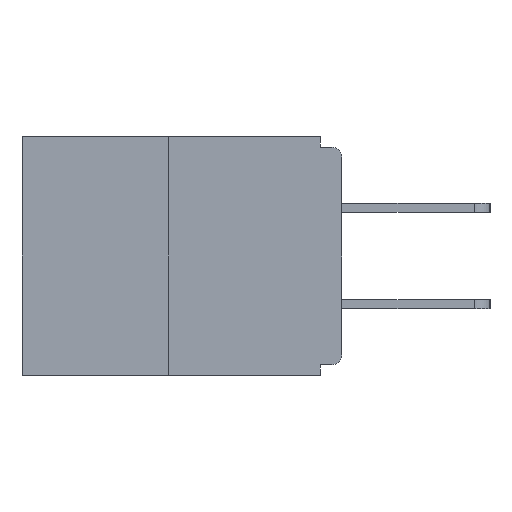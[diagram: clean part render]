
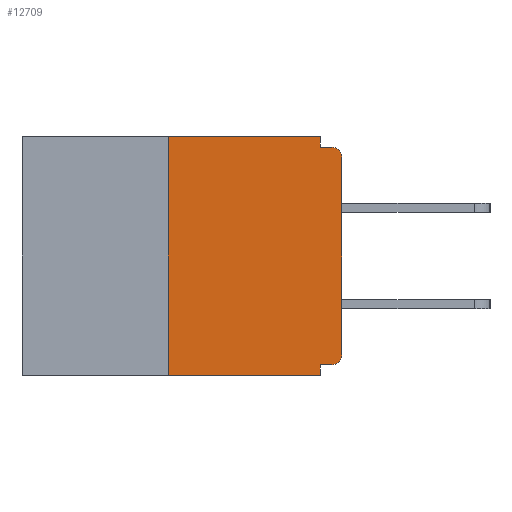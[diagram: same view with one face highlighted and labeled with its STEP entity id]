
A CAD part, left-side view. The second image highlights one B-rep face of the part: STEP entity #12709.
In plain terms, the highlighted planar face has unit normal (-1, 0, 0).
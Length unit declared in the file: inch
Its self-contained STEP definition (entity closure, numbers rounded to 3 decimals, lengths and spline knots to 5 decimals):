
#410 = VERTEX_POINT ( 'NONE', #9253 ) ;
#653 = CARTESIAN_POINT ( 'NONE',  ( 0., 0.25, 0. ) ) ;
#848 = CARTESIAN_POINT ( 'NONE',  ( 0., 0.031, -0.328 ) ) ;
#2643 = DIRECTION ( 'NONE',  ( 0., 0., 1. ) ) ;
#3361 = CARTESIAN_POINT ( 'NONE',  ( 0., 0.25, -0.343 ) ) ;
#3459 = CARTESIAN_POINT ( 'NONE',  ( 0., 0.46, 0. ) ) ;
#4541 = CARTESIAN_POINT ( 'NONE',  ( 0., 0.015, -0.03 ) ) ;
#4756 = CARTESIAN_POINT ( 'NONE',  ( 0., 0., -0.03 ) ) ;
#5009 = EDGE_CURVE ( 'NONE', #21462, #10018, #9504, .T. ) ;
#5322 = LINE ( 'NONE', #5993, #16218 ) ;
#5693 = CARTESIAN_POINT ( 'NONE',  ( 0., 0.031, 0. ) ) ;
#5720 = VERTEX_POINT ( 'NONE', #5693 ) ;
#5853 = DIRECTION ( 'NONE',  ( 0., 0., -1. ) ) ;
#5993 = CARTESIAN_POINT ( 'NONE',  ( 0., 0.031, -0.343 ) ) ;
#6022 = LINE ( 'NONE', #8962, #7115 ) ;
#6177 = LINE ( 'NONE', #7917, #17413 ) ;
#6811 = VERTEX_POINT ( 'NONE', #17372 ) ;
#6872 = EDGE_CURVE ( 'NONE', #9885, #410, #14978, .T. ) ;
#7115 = VECTOR ( 'NONE', #2643, 39.37008 ) ;
#7177 = ORIENTED_EDGE ( 'NONE', *, *, #23839, .T. ) ;
#7222 = ORIENTED_EDGE ( 'NONE', *, *, #8979, .F. ) ;
#7246 = CARTESIAN_POINT ( 'NONE',  ( 0., 0., -0.015 ) ) ;
#7917 = CARTESIAN_POINT ( 'NONE',  ( 0., 0.031, 0. ) ) ;
#8712 = VECTOR ( 'NONE', #20625, 39.37008 ) ;
#8740 = CIRCLE ( 'NONE', #18143, 0.015 ) ;
#8849 = DIRECTION ( 'NONE',  ( 0., -1., 0. ) ) ;
#8962 = CARTESIAN_POINT ( 'NONE',  ( 0., 0.25, 0. ) ) ;
#8979 = EDGE_CURVE ( 'NONE', #28953, #5720, #11420, .T. ) ;
#9055 = DIRECTION ( 'NONE',  ( 0., 0., -1. ) ) ;
#9080 = DIRECTION ( 'NONE',  ( -1., 0., 0. ) ) ;
#9253 = CARTESIAN_POINT ( 'NONE',  ( 0., 0.031, -0.343 ) ) ;
#9504 = CIRCLE ( 'NONE', #20768, 0.015 ) ;
#9885 = VERTEX_POINT ( 'NONE', #3361 ) ;
#10018 = VERTEX_POINT ( 'NONE', #20352 ) ;
#10610 = EDGE_LOOP ( 'NONE', ( #7222, #22445, #24540, #17256, #17356, #27365, #7177, #24020, #20868, #10907 ) ) ;
#10735 = FACE_OUTER_BOUND ( 'NONE', #10610, .T. ) ;
#10907 = ORIENTED_EDGE ( 'NONE', *, *, #12396, .F. ) ;
#11164 = VECTOR ( 'NONE', #12757, 39.37008 ) ;
#11420 = LINE ( 'NONE', #22328, #19164 ) ;
#11490 = CARTESIAN_POINT ( 'NONE',  ( 0., 0., -0.328 ) ) ;
#12235 = EDGE_CURVE ( 'NONE', #14406, #16925, #14967, .T. ) ;
#12396 = EDGE_CURVE ( 'NONE', #5720, #6811, #6177, .T. ) ;
#12709 = ADVANCED_FACE ( 'NONE', ( #10735 ), #15030, .F. ) ;
#12757 = DIRECTION ( 'NONE',  ( 0., -1., 0. ) ) ;
#13145 = VERTEX_POINT ( 'NONE', #27531 ) ;
#13376 = LINE ( 'NONE', #23783, #15107 ) ;
#13597 = LINE ( 'NONE', #7246, #25583 ) ;
#13974 = AXIS2_PLACEMENT_3D ( 'NONE', #3459, #17095, #28516 ) ;
#14406 = VERTEX_POINT ( 'NONE', #16720 ) ;
#14967 = LINE ( 'NONE', #11490, #8712 ) ;
#14978 = LINE ( 'NONE', #26286, #11164 ) ;
#15030 = PLANE ( 'NONE',  #13974 ) ;
#15107 = VECTOR ( 'NONE', #28446, 39.37008 ) ;
#16218 = VECTOR ( 'NONE', #21635, 39.37008 ) ;
#16720 = CARTESIAN_POINT ( 'NONE',  ( 0., 0.015, -0.328 ) ) ;
#16807 = EDGE_CURVE ( 'NONE', #9885, #28953, #6022, .T. ) ;
#16925 = VERTEX_POINT ( 'NONE', #848 ) ;
#17095 = DIRECTION ( 'NONE',  ( 1., 0., 0. ) ) ;
#17256 = ORIENTED_EDGE ( 'NONE', *, *, #17428, .F. ) ;
#17356 = ORIENTED_EDGE ( 'NONE', *, *, #12235, .F. ) ;
#17372 = CARTESIAN_POINT ( 'NONE',  ( 0., 0.031, -0.015 ) ) ;
#17413 = VECTOR ( 'NONE', #5853, 39.37008 ) ;
#17428 = EDGE_CURVE ( 'NONE', #16925, #410, #5322, .T. ) ;
#18143 = AXIS2_PLACEMENT_3D ( 'NONE', #20159, #22522, #9055 ) ;
#19164 = VECTOR ( 'NONE', #8849, 39.37008 ) ;
#20040 = EDGE_CURVE ( 'NONE', #14406, #13145, #8740, .T. ) ;
#20082 = DIRECTION ( 'NONE',  ( 0., 0., -1. ) ) ;
#20159 = CARTESIAN_POINT ( 'NONE',  ( 0., 0.015, -0.313 ) ) ;
#20352 = CARTESIAN_POINT ( 'NONE',  ( 0., 0.015, -0.015 ) ) ;
#20625 = DIRECTION ( 'NONE',  ( 0., 1., 0. ) ) ;
#20768 = AXIS2_PLACEMENT_3D ( 'NONE', #4541, #9080, #20082 ) ;
#20868 = ORIENTED_EDGE ( 'NONE', *, *, #26588, .F. ) ;
#21462 = VERTEX_POINT ( 'NONE', #4756 ) ;
#21635 = DIRECTION ( 'NONE',  ( 0., 0., -1. ) ) ;
#22328 = CARTESIAN_POINT ( 'NONE',  ( 0., 0.46, 0. ) ) ;
#22445 = ORIENTED_EDGE ( 'NONE', *, *, #16807, .F. ) ;
#22522 = DIRECTION ( 'NONE',  ( -1., 0., 0. ) ) ;
#23783 = CARTESIAN_POINT ( 'NONE',  ( 0., 0., 0. ) ) ;
#23839 = EDGE_CURVE ( 'NONE', #13145, #21462, #13376, .T. ) ;
#24020 = ORIENTED_EDGE ( 'NONE', *, *, #5009, .T. ) ;
#24540 = ORIENTED_EDGE ( 'NONE', *, *, #6872, .T. ) ;
#25583 = VECTOR ( 'NONE', #27830, 39.37008 ) ;
#26286 = CARTESIAN_POINT ( 'NONE',  ( 0., 0.46, -0.343 ) ) ;
#26588 = EDGE_CURVE ( 'NONE', #6811, #10018, #13597, .T. ) ;
#27365 = ORIENTED_EDGE ( 'NONE', *, *, #20040, .T. ) ;
#27531 = CARTESIAN_POINT ( 'NONE',  ( 0., 0., -0.313 ) ) ;
#27830 = DIRECTION ( 'NONE',  ( 0., -1., 0. ) ) ;
#28446 = DIRECTION ( 'NONE',  ( 0., 0., 1. ) ) ;
#28516 = DIRECTION ( 'NONE',  ( 0., 0., -1. ) ) ;
#28953 = VERTEX_POINT ( 'NONE', #653 ) ;
